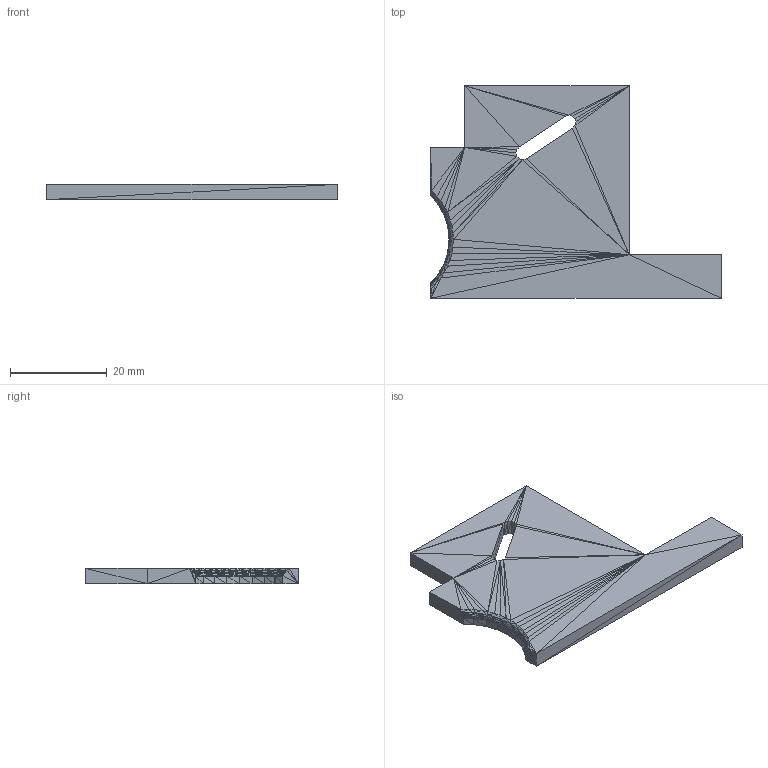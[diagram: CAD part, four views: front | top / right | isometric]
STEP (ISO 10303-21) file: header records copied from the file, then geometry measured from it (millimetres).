
FILE_DESCRIPTION(('FreeCAD Model'),'2;1');
FILE_NAME('Open CASCADE Shape Model','2021-09-30T12:02:18',('Author'),( ''),'Open CASCADE STEP processor 7.4','FreeCAD','Unknown');
FILE_SCHEMA(('AUTOMOTIVE_DESIGN { 1 0 10303 214 1 1 1 1 }'));
Length unit declared in the file: millimetre
Products named in the file (1): Trigger_Left001_(Solid)
Bounding box: 60.07 x 43.94 x 3.17 mm (x, y, z)
Volume: 5698.3 mm3; surface area: 4352.6 mm2
Topology: 1 solids, 1 shells, 312 faces, 468 edges, 156 vertices
Faces by surface type: plane 312
Entity records: 11730 total; most frequent: CARTESIAN_POINT 2341, DIRECTION 1562, ORIENTED_EDGE 936, LINE 936, VECTOR 936, PCURVE 936, DEFINITIONAL_REPRESENTATION 936, EDGE_CURVE 468
